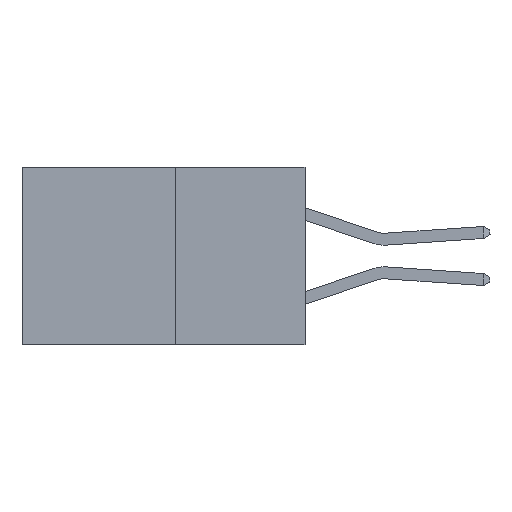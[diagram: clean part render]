
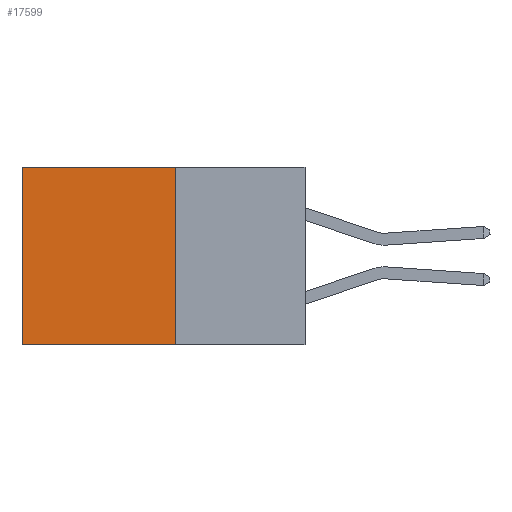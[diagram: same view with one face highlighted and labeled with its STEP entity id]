
A CAD part, left-side view. The second image highlights one B-rep face of the part: STEP entity #17599.
In plain terms, the highlighted planar face has unit normal (-1, 0, 0).
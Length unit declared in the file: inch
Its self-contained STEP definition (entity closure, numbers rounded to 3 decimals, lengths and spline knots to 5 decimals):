
#987 = EDGE_CURVE ( 'NONE', #15563, #2056, #14975, .T. ) ;
#2056 = VERTEX_POINT ( 'NONE', #4895 ) ;
#2240 = CARTESIAN_POINT ( 'NONE',  ( 0.277, 0.59, -0.37 ) ) ;
#2271 = DIRECTION ( 'NONE',  ( 0., 1., 0. ) ) ;
#2551 = DIRECTION ( 'NONE',  ( 0., 1., 0. ) ) ;
#2821 = VERTEX_POINT ( 'NONE', #18927 ) ;
#2964 = DIRECTION ( 'NONE',  ( 0., 0., -1. ) ) ;
#3045 = VERTEX_POINT ( 'NONE', #8166 ) ;
#3336 = VECTOR ( 'NONE', #2964, 39.37008 ) ;
#3428 = VECTOR ( 'NONE', #2271, 39.37008 ) ;
#4071 = VECTOR ( 'NONE', #9861, 39.37008 ) ;
#4131 = EDGE_LOOP ( 'NONE', ( #13645, #18315, #12497, #13035 ) ) ;
#4549 = AXIS2_PLACEMENT_3D ( 'NONE', #16759, #8032, #18214 ) ;
#4558 = CARTESIAN_POINT ( 'NONE',  ( 0.277, 0.59, 0. ) ) ;
#4895 = CARTESIAN_POINT ( 'NONE',  ( 0.277, 0.59, -0.37 ) ) ;
#5087 = PLANE ( 'NONE',  #4549 ) ;
#5925 = LINE ( 'NONE', #17190, #4071 ) ;
#6580 = FACE_OUTER_BOUND ( 'NONE', #4131, .T. ) ;
#7330 = VECTOR ( 'NONE', #2551, 39.37008 ) ;
#8032 = DIRECTION ( 'NONE',  ( 1., 0., 0. ) ) ;
#8166 = CARTESIAN_POINT ( 'NONE',  ( 0.277, 0.27, -0.37 ) ) ;
#9579 = CARTESIAN_POINT ( 'NONE',  ( 0.277, 0.27, 0. ) ) ;
#9861 = DIRECTION ( 'NONE',  ( 0., 0., -1. ) ) ;
#10719 = LINE ( 'NONE', #14244, #7330 ) ;
#11134 = EDGE_CURVE ( 'NONE', #2821, #3045, #5925, .T. ) ;
#12497 = ORIENTED_EDGE ( 'NONE', *, *, #11134, .F. ) ;
#13035 = ORIENTED_EDGE ( 'NONE', *, *, #18899, .T. ) ;
#13645 = ORIENTED_EDGE ( 'NONE', *, *, #987, .T. ) ;
#14244 = CARTESIAN_POINT ( 'NONE',  ( 0.277, 0.27, -0.37 ) ) ;
#14975 = LINE ( 'NONE', #2240, #3336 ) ;
#15073 = LINE ( 'NONE', #9579, #3428 ) ;
#15296 = EDGE_CURVE ( 'NONE', #3045, #2056, #10719, .T. ) ;
#15563 = VERTEX_POINT ( 'NONE', #4558 ) ;
#16759 = CARTESIAN_POINT ( 'NONE',  ( 0.277, 0.27, -0.37 ) ) ;
#17190 = CARTESIAN_POINT ( 'NONE',  ( 0.277, 0.27, -0.37 ) ) ;
#17599 = ADVANCED_FACE ( 'NONE', ( #6580 ), #5087, .F. ) ;
#18214 = DIRECTION ( 'NONE',  ( 0., 0., -1. ) ) ;
#18315 = ORIENTED_EDGE ( 'NONE', *, *, #15296, .F. ) ;
#18899 = EDGE_CURVE ( 'NONE', #2821, #15563, #15073, .T. ) ;
#18927 = CARTESIAN_POINT ( 'NONE',  ( 0.277, 0.27, 0. ) ) ;
